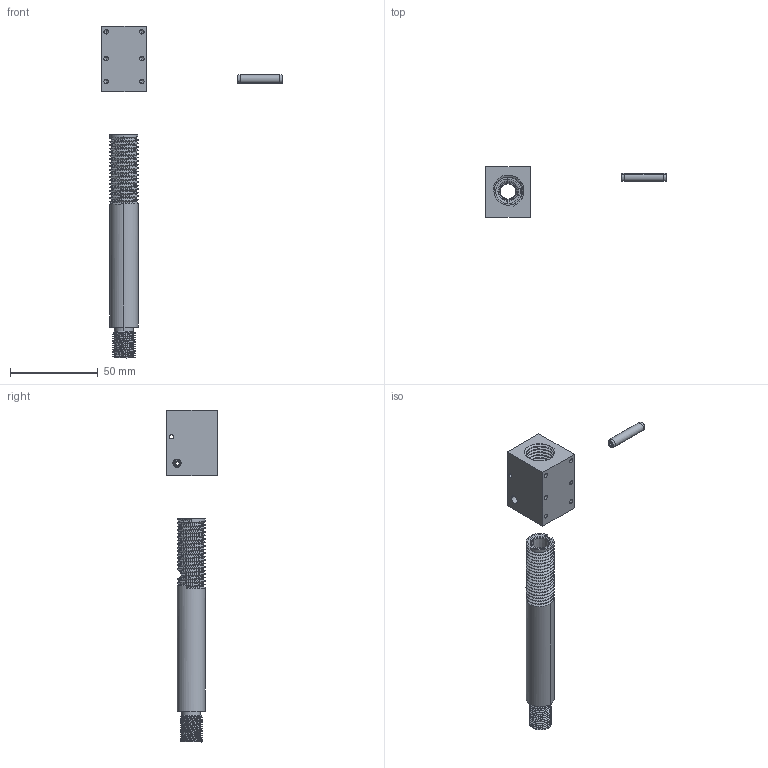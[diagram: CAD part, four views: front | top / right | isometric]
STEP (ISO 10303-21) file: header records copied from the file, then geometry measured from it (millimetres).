
FILE_DESCRIPTION (( 'STEP AP214' ), '1' );
FILE_NAME ('PPDW9 V4 ECM Barrel and block.STEP', '2020-12-31T18:43:36', ( '' ), ( '' ), 'SwSTEP 2.0', 'SolidWorks 2020', '' );
FILE_SCHEMA (( 'AUTOMOTIVE_DESIGN' ));
Length unit declared in the file: inch
Products named in the file (4): Barrel spring pin 95755A324_95755A324; PPDW9 V4 ECM Barrel and block; V4 9mm Barrel block ECM; Barrel PPDW9  V3-V4 ECM barrel
Assembly tree (3 placements, depth 2):
  PPDW9 V4 ECM Barrel and block
    V4 9mm Barrel block ECM
    Barrel PPDW9  V3-V4 ECM barrel
    Barrel spring pin 95755A324_95755A324
Bounding box: 102.69 x 28.7 x 188.65 mm (x, y, z)
Volume: 33052.4 mm3; surface area: 21613.7 mm2
Topology: 3 solids, 3 shells, 210 faces, 599 edges, 388 vertices
Faces by surface type: cylinder 138, cone 24, bspline 22, plane 22, torus 4
Entity records: 29226 total; most frequent: CARTESIAN_POINT 24227, ORIENTED_EDGE 1174, DIRECTION 785, EDGE_CURVE 587, VERTEX_POINT 388, AXIS2_PLACEMENT_3D 299, EDGE_LOOP 225, ADVANCED_FACE 210
